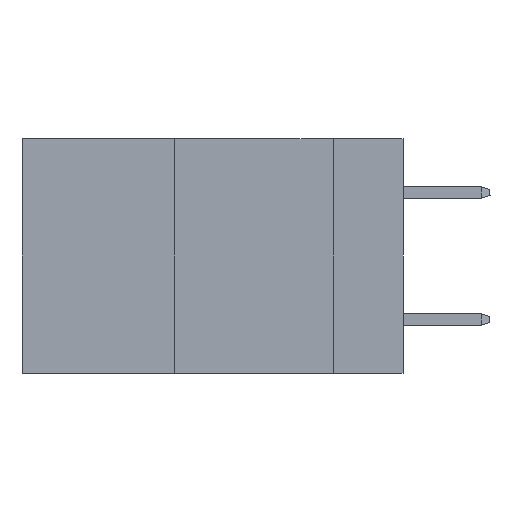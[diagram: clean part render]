
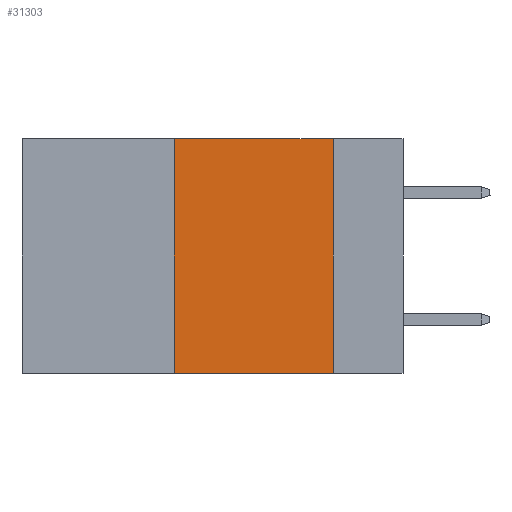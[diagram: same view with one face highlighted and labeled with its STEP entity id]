
A CAD part, left-side view. The second image highlights one B-rep face of the part: STEP entity #31303.
In plain terms, the highlighted planar face has unit normal (-1, 0, 0).
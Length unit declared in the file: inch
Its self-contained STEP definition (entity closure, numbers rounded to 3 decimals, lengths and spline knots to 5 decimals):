
#556 = CARTESIAN_POINT ( 'NONE',  ( 0., 0.11, -0.37 ) ) ;
#578 = VECTOR ( 'NONE', #12834, 39.37008 ) ;
#3487 = CARTESIAN_POINT ( 'NONE',  ( 0., 0.36, 0. ) ) ;
#4278 = VERTEX_POINT ( 'NONE', #556 ) ;
#9195 = CARTESIAN_POINT ( 'NONE',  ( 0., 0.6, 0. ) ) ;
#9477 = CARTESIAN_POINT ( 'NONE',  ( 0., 0.6, 0. ) ) ;
#10187 = VERTEX_POINT ( 'NONE', #3487 ) ;
#10303 = CARTESIAN_POINT ( 'NONE',  ( 0., 0.11, 0. ) ) ;
#11409 = VECTOR ( 'NONE', #23839, 39.37008 ) ;
#11834 = ORIENTED_EDGE ( 'NONE', *, *, #41692, .F. ) ;
#12834 = DIRECTION ( 'NONE',  ( 0., 0., -1. ) ) ;
#12882 = VECTOR ( 'NONE', #15677, 39.37008 ) ;
#15677 = DIRECTION ( 'NONE',  ( 0., -1., 0. ) ) ;
#15740 = DIRECTION ( 'NONE',  ( 0., 0., -1. ) ) ;
#15904 = LINE ( 'NONE', #9195, #42184 ) ;
#17276 = EDGE_CURVE ( 'NONE', #37678, #4278, #22262, .T. ) ;
#19222 = ORIENTED_EDGE ( 'NONE', *, *, #17276, .F. ) ;
#20703 = CARTESIAN_POINT ( 'NONE',  ( 0., 0.36, 0. ) ) ;
#22262 = LINE ( 'NONE', #39446, #578 ) ;
#23839 = DIRECTION ( 'NONE',  ( 0., 0., 1. ) ) ;
#27652 = AXIS2_PLACEMENT_3D ( 'NONE', #9477, #36765, #15740 ) ;
#29550 = VERTEX_POINT ( 'NONE', #44055 ) ;
#30291 = PLANE ( 'NONE',  #27652 ) ;
#31303 = ADVANCED_FACE ( 'NONE', ( #32965 ), #30291, .F. ) ;
#32965 = FACE_OUTER_BOUND ( 'NONE', #41429, .T. ) ;
#34192 = ORIENTED_EDGE ( 'NONE', *, *, #36667, .F. ) ;
#35415 = ORIENTED_EDGE ( 'NONE', *, *, #41718, .T. ) ;
#36495 = DIRECTION ( 'NONE',  ( 0., -1., 0. ) ) ;
#36667 = EDGE_CURVE ( 'NONE', #29550, #10187, #41497, .T. ) ;
#36704 = LINE ( 'NONE', #42996, #12882 ) ;
#36765 = DIRECTION ( 'NONE',  ( 1., 0., 0. ) ) ;
#37678 = VERTEX_POINT ( 'NONE', #10303 ) ;
#39446 = CARTESIAN_POINT ( 'NONE',  ( 0., 0.11, 0. ) ) ;
#41429 = EDGE_LOOP ( 'NONE', ( #19222, #11834, #34192, #35415 ) ) ;
#41497 = LINE ( 'NONE', #20703, #11409 ) ;
#41692 = EDGE_CURVE ( 'NONE', #10187, #37678, #15904, .T. ) ;
#41718 = EDGE_CURVE ( 'NONE', #29550, #4278, #36704, .T. ) ;
#42184 = VECTOR ( 'NONE', #36495, 39.37008 ) ;
#42996 = CARTESIAN_POINT ( 'NONE',  ( 0., 0.6, -0.37 ) ) ;
#44055 = CARTESIAN_POINT ( 'NONE',  ( 0., 0.36, -0.37 ) ) ;
